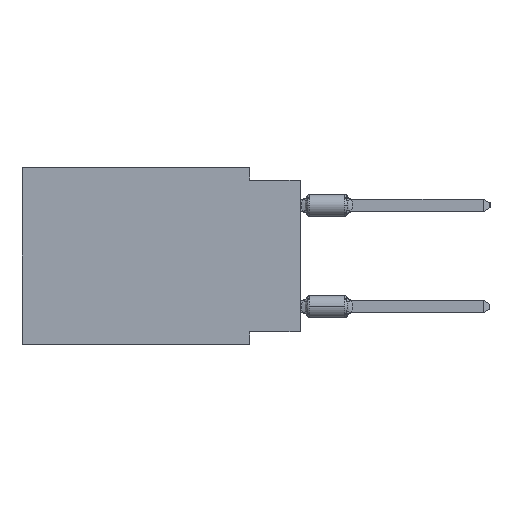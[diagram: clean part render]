
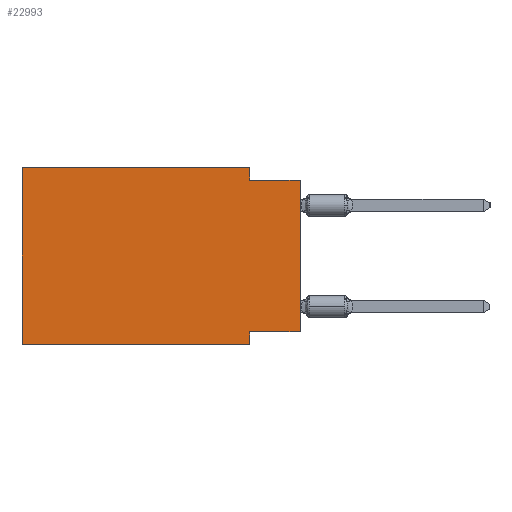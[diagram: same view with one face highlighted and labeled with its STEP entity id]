
A CAD part, left-side view. The second image highlights one B-rep face of the part: STEP entity #22993.
In plain terms, the highlighted planar face has unit normal (-1, 0, 0).
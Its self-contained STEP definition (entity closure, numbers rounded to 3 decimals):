
#138 = AXIS2_PLACEMENT_3D ( 'NONE', #9271, #23502, #51023 ) ;
#1006 = LINE ( 'NONE', #19195, #6598 ) ;
#1070 = DIRECTION ( 'NONE',  ( 0., -1., 0. ) ) ;
#1461 = CARTESIAN_POINT ( 'NONE',  ( 0., 13.97, 0. ) ) ;
#2270 = LINE ( 'NONE', #34374, #3959 ) ;
#2585 = LINE ( 'NONE', #20780, #4979 ) ;
#3555 = VECTOR ( 'NONE', #5039, 1000. ) ;
#3959 = VECTOR ( 'NONE', #1070, 1000. ) ;
#4072 = DIRECTION ( 'NONE',  ( 0., 0., 1. ) ) ;
#4965 = EDGE_CURVE ( 'NONE', #7177, #33404, #24431, .T. ) ;
#4979 = VECTOR ( 'NONE', #57689, 1000. ) ;
#5039 = DIRECTION ( 'NONE',  ( 0., 1., 0. ) ) ;
#5612 = LINE ( 'NONE', #16212, #20442 ) ;
#6430 = EDGE_LOOP ( 'NONE', ( #25792, #46954, #22184, #39128, #48697, #41110, #55083, #18131 ) ) ;
#6434 = CARTESIAN_POINT ( 'NONE',  ( 0., 0., -0.635 ) ) ;
#6598 = VECTOR ( 'NONE', #9798, 1000. ) ;
#7177 = VERTEX_POINT ( 'NONE', #57272 ) ;
#8420 = EDGE_CURVE ( 'NONE', #51065, #33156, #5612, .T. ) ;
#9271 = CARTESIAN_POINT ( 'NONE',  ( 0., 13.97, 0. ) ) ;
#9798 = DIRECTION ( 'NONE',  ( 0., -1., 0. ) ) ;
#9897 = CARTESIAN_POINT ( 'NONE',  ( 0., 2.54, 0. ) ) ;
#11637 = EDGE_CURVE ( 'NONE', #7177, #15024, #40713, .T. ) ;
#12025 = CARTESIAN_POINT ( 'NONE',  ( 0., 2.54, -8.89 ) ) ;
#12341 = LINE ( 'NONE', #12025, #17007 ) ;
#14106 = PLANE ( 'NONE',  #138 ) ;
#15024 = VERTEX_POINT ( 'NONE', #6434 ) ;
#15532 = VECTOR ( 'NONE', #33940, 1000. ) ;
#15692 = CARTESIAN_POINT ( 'NONE',  ( 0., 2.54, -8.255 ) ) ;
#16135 = CARTESIAN_POINT ( 'NONE',  ( 0., 2.54, -0.635 ) ) ;
#16212 = CARTESIAN_POINT ( 'NONE',  ( 0., 13.97, 0. ) ) ;
#17007 = VECTOR ( 'NONE', #57750, 1000. ) ;
#18131 = ORIENTED_EDGE ( 'NONE', *, *, #4965, .F. ) ;
#19105 = VERTEX_POINT ( 'NONE', #54646 ) ;
#19195 = CARTESIAN_POINT ( 'NONE',  ( 0., 0., -0.635 ) ) ;
#20040 = LINE ( 'NONE', #38482, #15532 ) ;
#20442 = VECTOR ( 'NONE', #38895, 1000. ) ;
#20597 = VERTEX_POINT ( 'NONE', #16135 ) ;
#20780 = CARTESIAN_POINT ( 'NONE',  ( 0., 2.54, 0. ) ) ;
#21958 = EDGE_CURVE ( 'NONE', #33156, #49872, #2270, .T. ) ;
#22184 = ORIENTED_EDGE ( 'NONE', *, *, #37921, .F. ) ;
#22993 = ADVANCED_FACE ( 'NONE', ( #28648 ), #14106, .F. ) ;
#23502 = DIRECTION ( 'NONE',  ( 1., 0., 0. ) ) ;
#24392 = VECTOR ( 'NONE', #4072, 1000. ) ;
#24431 = LINE ( 'NONE', #51059, #3555 ) ;
#25792 = ORIENTED_EDGE ( 'NONE', *, *, #11637, .T. ) ;
#28648 = FACE_OUTER_BOUND ( 'NONE', #6430, .T. ) ;
#29278 = CARTESIAN_POINT ( 'NONE',  ( 0., 13.97, -8.89 ) ) ;
#33156 = VERTEX_POINT ( 'NONE', #1461 ) ;
#33404 = VERTEX_POINT ( 'NONE', #15692 ) ;
#33940 = DIRECTION ( 'NONE',  ( 0., -1., 0. ) ) ;
#34045 = EDGE_CURVE ( 'NONE', #20597, #15024, #1006, .T. ) ;
#34374 = CARTESIAN_POINT ( 'NONE',  ( 0., 13.97, 0. ) ) ;
#34679 = EDGE_CURVE ( 'NONE', #51065, #19105, #20040, .T. ) ;
#37921 = EDGE_CURVE ( 'NONE', #49872, #20597, #2585, .T. ) ;
#38482 = CARTESIAN_POINT ( 'NONE',  ( 0., 13.97, -8.89 ) ) ;
#38895 = DIRECTION ( 'NONE',  ( 0., 0., 1. ) ) ;
#39128 = ORIENTED_EDGE ( 'NONE', *, *, #21958, .F. ) ;
#40713 = LINE ( 'NONE', #45548, #24392 ) ;
#41110 = ORIENTED_EDGE ( 'NONE', *, *, #34679, .T. ) ;
#45548 = CARTESIAN_POINT ( 'NONE',  ( 0., 0., 0. ) ) ;
#46954 = ORIENTED_EDGE ( 'NONE', *, *, #34045, .F. ) ;
#48697 = ORIENTED_EDGE ( 'NONE', *, *, #8420, .F. ) ;
#49872 = VERTEX_POINT ( 'NONE', #9897 ) ;
#51023 = DIRECTION ( 'NONE',  ( 0., 0., -1. ) ) ;
#51059 = CARTESIAN_POINT ( 'NONE',  ( 0., 0., -8.255 ) ) ;
#51065 = VERTEX_POINT ( 'NONE', #29278 ) ;
#54646 = CARTESIAN_POINT ( 'NONE',  ( 0., 2.54, -8.89 ) ) ;
#55083 = ORIENTED_EDGE ( 'NONE', *, *, #56934, .F. ) ;
#56934 = EDGE_CURVE ( 'NONE', #33404, #19105, #12341, .T. ) ;
#57272 = CARTESIAN_POINT ( 'NONE',  ( 0., 0., -8.255 ) ) ;
#57689 = DIRECTION ( 'NONE',  ( 0., 0., -1. ) ) ;
#57750 = DIRECTION ( 'NONE',  ( 0., 0., -1. ) ) ;
